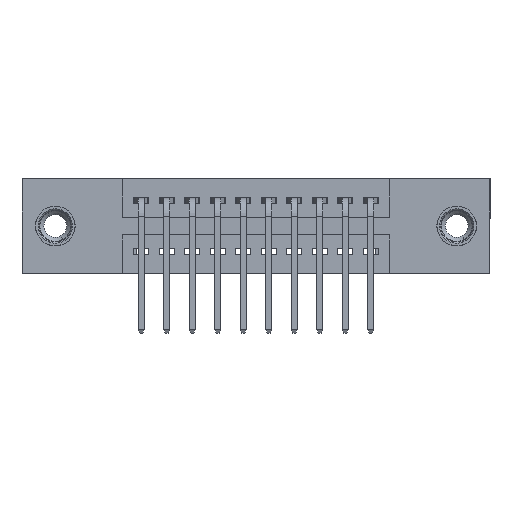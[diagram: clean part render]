
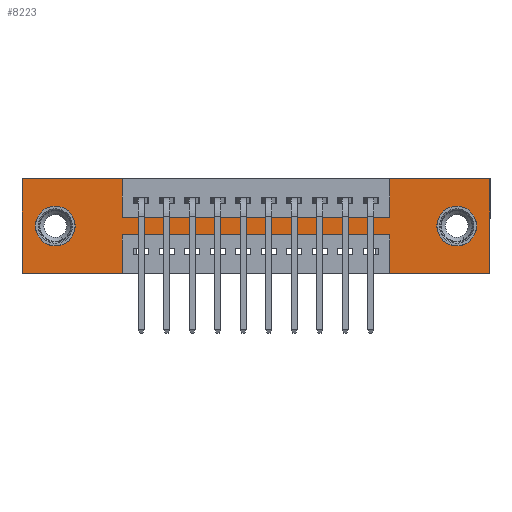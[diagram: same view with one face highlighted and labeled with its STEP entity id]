
A CAD part, front view. The second image highlights one B-rep face of the part: STEP entity #8223.
In plain terms, the highlighted planar face has unit normal (0, -1, 0).
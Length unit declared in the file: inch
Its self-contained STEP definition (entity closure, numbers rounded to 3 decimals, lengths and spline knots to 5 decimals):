
#67 = EDGE_CURVE ( 'NONE', #1339, #11391, #10440, .T. ) ;
#156 = CARTESIAN_POINT ( 'NONE',  ( 0.13, 0., -0.185 ) ) ;
#175 = LINE ( 'NONE', #6462, #6114 ) ;
#178 = CARTESIAN_POINT ( 'NONE',  ( 0.3925, 0., -0.15 ) ) ;
#489 = LINE ( 'NONE', #2541, #10583 ) ;
#529 = EDGE_CURVE ( 'NONE', #3014, #15972, #14744, .T. ) ;
#532 = CARTESIAN_POINT ( 'NONE',  ( 0.3925, 0., -0.37 ) ) ;
#799 = EDGE_LOOP ( 'NONE', ( #4511, #5727 ) ) ;
#966 = DIRECTION ( 'NONE',  ( 0., 0., 1. ) ) ;
#1264 = ORIENTED_EDGE ( 'NONE', *, *, #6913, .F. ) ;
#1339 = VERTEX_POINT ( 'NONE', #8443 ) ;
#1529 = DIRECTION ( 'NONE',  ( 0., 0., 1. ) ) ;
#1613 = CARTESIAN_POINT ( 'NONE',  ( 0., 0., 0. ) ) ;
#1901 = CARTESIAN_POINT ( 'NONE',  ( 1.4425, 0., -0.37 ) ) ;
#1910 = VERTEX_POINT ( 'NONE', #16460 ) ;
#1972 = EDGE_CURVE ( 'NONE', #15239, #2519, #2862, .T. ) ;
#2015 = CIRCLE ( 'NONE', #12170, 0.078 ) ;
#2458 = CARTESIAN_POINT ( 'NONE',  ( 0., 0., -0.37 ) ) ;
#2519 = VERTEX_POINT ( 'NONE', #4449 ) ;
#2522 = LINE ( 'NONE', #12769, #15750 ) ;
#2536 = CARTESIAN_POINT ( 'NONE',  ( 1.4425, 0., 0. ) ) ;
#2541 = CARTESIAN_POINT ( 'NONE',  ( 0.3925, 0., -0.15 ) ) ;
#2862 = LINE ( 'NONE', #7168, #9425 ) ;
#2865 = CARTESIAN_POINT ( 'NONE',  ( 1.705, 0., -0.107 ) ) ;
#2927 = LINE ( 'NONE', #9059, #9486 ) ;
#3014 = VERTEX_POINT ( 'NONE', #2458 ) ;
#3538 = CARTESIAN_POINT ( 'NONE',  ( 0.3925, 0., 0. ) ) ;
#3755 = EDGE_CURVE ( 'NONE', #11391, #9415, #10949, .T. ) ;
#4160 = VECTOR ( 'NONE', #13071, 39.37008 ) ;
#4161 = CARTESIAN_POINT ( 'NONE',  ( 0.3925, 0., -0.22 ) ) ;
#4449 = CARTESIAN_POINT ( 'NONE',  ( 1.835, 0., 0. ) ) ;
#4511 = ORIENTED_EDGE ( 'NONE', *, *, #8137, .T. ) ;
#4864 = CARTESIAN_POINT ( 'NONE',  ( 0., 0., -0.37 ) ) ;
#4930 = DIRECTION ( 'NONE',  ( 0., 0., -1. ) ) ;
#5026 = AXIS2_PLACEMENT_3D ( 'NONE', #156, #9443, #1529 ) ;
#5072 = VECTOR ( 'NONE', #5987, 39.37008 ) ;
#5142 = ORIENTED_EDGE ( 'NONE', *, *, #6101, .F. ) ;
#5353 = ORIENTED_EDGE ( 'NONE', *, *, #16474, .F. ) ;
#5378 = EDGE_LOOP ( 'NONE', ( #9885, #6919, #7741, #5142, #8521, #5543, #15941, #16689, #14219, #1264, #8336, #5353 ) ) ;
#5523 = ORIENTED_EDGE ( 'NONE', *, *, #10659, .T. ) ;
#5543 = ORIENTED_EDGE ( 'NONE', *, *, #1972, .F. ) ;
#5727 = ORIENTED_EDGE ( 'NONE', *, *, #14729, .T. ) ;
#5987 = DIRECTION ( 'NONE',  ( 0., 0., 1. ) ) ;
#6001 = CARTESIAN_POINT ( 'NONE',  ( 0.13, 0., -0.185 ) ) ;
#6031 = CIRCLE ( 'NONE', #13560, 0.078 ) ;
#6101 = EDGE_CURVE ( 'NONE', #10907, #1339, #16678, .T. ) ;
#6114 = VECTOR ( 'NONE', #9019, 39.37008 ) ;
#6422 = EDGE_CURVE ( 'NONE', #9415, #15403, #175, .T. ) ;
#6434 = CARTESIAN_POINT ( 'NONE',  ( 0.3925, 0., 0. ) ) ;
#6462 = CARTESIAN_POINT ( 'NONE',  ( 0.3925, 0., -0.37 ) ) ;
#6698 = CARTESIAN_POINT ( 'NONE',  ( 0., 0., 0. ) ) ;
#6738 = EDGE_CURVE ( 'NONE', #10102, #13054, #12222, .T. ) ;
#6744 = CARTESIAN_POINT ( 'NONE',  ( 1.705, 0., -0.185 ) ) ;
#6764 = CARTESIAN_POINT ( 'NONE',  ( 1.705, 0., -0.185 ) ) ;
#6913 = EDGE_CURVE ( 'NONE', #15972, #10102, #2927, .T. ) ;
#6919 = ORIENTED_EDGE ( 'NONE', *, *, #3755, .F. ) ;
#7036 = FACE_OUTER_BOUND ( 'NONE', #5378, .T. ) ;
#7079 = DIRECTION ( 'NONE',  ( -1., 0., 0. ) ) ;
#7083 = VECTOR ( 'NONE', #966, 39.37008 ) ;
#7168 = CARTESIAN_POINT ( 'NONE',  ( 0., 0., 0. ) ) ;
#7203 = VERTEX_POINT ( 'NONE', #9606 ) ;
#7281 = DIRECTION ( 'NONE',  ( 0., 0., 1. ) ) ;
#7375 = VERTEX_POINT ( 'NONE', #16220 ) ;
#7451 = DIRECTION ( 'NONE',  ( 0., 0., -1. ) ) ;
#7741 = ORIENTED_EDGE ( 'NONE', *, *, #67, .F. ) ;
#8038 = DIRECTION ( 'NONE',  ( 0., 0., -1. ) ) ;
#8056 = DIRECTION ( 'NONE',  ( 0., 0., -1. ) ) ;
#8137 = EDGE_CURVE ( 'NONE', #7375, #1910, #2015, .T. ) ;
#8223 = ADVANCED_FACE ( 'NONE', ( #14527, #13733, #7036 ), #12388, .T. ) ;
#8283 = CARTESIAN_POINT ( 'NONE',  ( 1.4425, 0., -0.22 ) ) ;
#8336 = ORIENTED_EDGE ( 'NONE', *, *, #529, .F. ) ;
#8443 = CARTESIAN_POINT ( 'NONE',  ( 1.4425, 0., -0.37 ) ) ;
#8453 = EDGE_CURVE ( 'NONE', #13054, #7203, #489, .T. ) ;
#8521 = ORIENTED_EDGE ( 'NONE', *, *, #12241, .F. ) ;
#8522 = EDGE_CURVE ( 'NONE', #8973, #16376, #6031, .T. ) ;
#8723 = VECTOR ( 'NONE', #14192, 39.37008 ) ;
#8835 = AXIS2_PLACEMENT_3D ( 'NONE', #6744, #15519, #8038 ) ;
#8892 = VECTOR ( 'NONE', #4930, 39.37008 ) ;
#8973 = VERTEX_POINT ( 'NONE', #13958 ) ;
#9019 = DIRECTION ( 'NONE',  ( 0., 0., -1. ) ) ;
#9059 = CARTESIAN_POINT ( 'NONE',  ( 0., 0., 0. ) ) ;
#9415 = VERTEX_POINT ( 'NONE', #12687 ) ;
#9425 = VECTOR ( 'NONE', #15916, 39.37008 ) ;
#9443 = DIRECTION ( 'NONE',  ( 0., 1., 0. ) ) ;
#9486 = VECTOR ( 'NONE', #14049, 39.37008 ) ;
#9540 = VECTOR ( 'NONE', #12276, 39.37008 ) ;
#9606 = CARTESIAN_POINT ( 'NONE',  ( 1.4425, 0., -0.15 ) ) ;
#9885 = ORIENTED_EDGE ( 'NONE', *, *, #6422, .F. ) ;
#9900 = LINE ( 'NONE', #2536, #8723 ) ;
#10102 = VERTEX_POINT ( 'NONE', #6434 ) ;
#10288 = DIRECTION ( 'NONE',  ( 0., 0., -1. ) ) ;
#10353 = DIRECTION ( 'NONE',  ( 1., 0., 0. ) ) ;
#10440 = LINE ( 'NONE', #1901, #7083 ) ;
#10569 = CIRCLE ( 'NONE', #5026, 0.078 ) ;
#10583 = VECTOR ( 'NONE', #10353, 39.37008 ) ;
#10659 = EDGE_CURVE ( 'NONE', #16376, #8973, #15230, .T. ) ;
#10907 = VERTEX_POINT ( 'NONE', #14773 ) ;
#10949 = LINE ( 'NONE', #4161, #4160 ) ;
#11391 = VERTEX_POINT ( 'NONE', #8283 ) ;
#11796 = EDGE_CURVE ( 'NONE', #7203, #15239, #9900, .T. ) ;
#12170 = AXIS2_PLACEMENT_3D ( 'NONE', #6001, #14812, #7281 ) ;
#12222 = LINE ( 'NONE', #3538, #8892 ) ;
#12241 = EDGE_CURVE ( 'NONE', #2519, #10907, #2522, .T. ) ;
#12276 = DIRECTION ( 'NONE',  ( -1., 0., 0. ) ) ;
#12388 = PLANE ( 'NONE',  #16315 ) ;
#12625 = ORIENTED_EDGE ( 'NONE', *, *, #8522, .T. ) ;
#12687 = CARTESIAN_POINT ( 'NONE',  ( 0.3925, 0., -0.22 ) ) ;
#12769 = CARTESIAN_POINT ( 'NONE',  ( 1.835, 0., 0. ) ) ;
#13054 = VERTEX_POINT ( 'NONE', #178 ) ;
#13071 = DIRECTION ( 'NONE',  ( -1., 0., 0. ) ) ;
#13437 = VECTOR ( 'NONE', #7079, 39.37008 ) ;
#13472 = EDGE_LOOP ( 'NONE', ( #5523, #12625 ) ) ;
#13558 = CARTESIAN_POINT ( 'NONE',  ( 0., 0., -0.37 ) ) ;
#13560 = AXIS2_PLACEMENT_3D ( 'NONE', #6764, #15539, #8056 ) ;
#13733 = FACE_BOUND ( 'NONE', #799, .T. ) ;
#13958 = CARTESIAN_POINT ( 'NONE',  ( 1.705, 0., -0.263 ) ) ;
#14049 = DIRECTION ( 'NONE',  ( 1., 0., 0. ) ) ;
#14192 = DIRECTION ( 'NONE',  ( 0., 0., 1. ) ) ;
#14219 = ORIENTED_EDGE ( 'NONE', *, *, #6738, .F. ) ;
#14527 = FACE_BOUND ( 'NONE', #13472, .T. ) ;
#14621 = CARTESIAN_POINT ( 'NONE',  ( 0., 0., -0.37 ) ) ;
#14729 = EDGE_CURVE ( 'NONE', #1910, #7375, #10569, .T. ) ;
#14744 = LINE ( 'NONE', #6698, #5072 ) ;
#14773 = CARTESIAN_POINT ( 'NONE',  ( 1.835, 0., -0.37 ) ) ;
#14812 = DIRECTION ( 'NONE',  ( 0., 1., 0. ) ) ;
#14958 = DIRECTION ( 'NONE',  ( 0., -1., 0. ) ) ;
#15230 = CIRCLE ( 'NONE', #8835, 0.078 ) ;
#15239 = VERTEX_POINT ( 'NONE', #15786 ) ;
#15403 = VERTEX_POINT ( 'NONE', #532 ) ;
#15519 = DIRECTION ( 'NONE',  ( 0., 1., 0. ) ) ;
#15539 = DIRECTION ( 'NONE',  ( 0., 1., 0. ) ) ;
#15750 = VECTOR ( 'NONE', #10288, 39.37008 ) ;
#15786 = CARTESIAN_POINT ( 'NONE',  ( 1.4425, 0., 0. ) ) ;
#15916 = DIRECTION ( 'NONE',  ( 1., 0., 0. ) ) ;
#15941 = ORIENTED_EDGE ( 'NONE', *, *, #11796, .F. ) ;
#15972 = VERTEX_POINT ( 'NONE', #1613 ) ;
#16145 = LINE ( 'NONE', #13558, #9540 ) ;
#16220 = CARTESIAN_POINT ( 'NONE',  ( 0.13, 0., -0.107 ) ) ;
#16315 = AXIS2_PLACEMENT_3D ( 'NONE', #4864, #14958, #7451 ) ;
#16376 = VERTEX_POINT ( 'NONE', #2865 ) ;
#16460 = CARTESIAN_POINT ( 'NONE',  ( 0.13, 0., -0.263 ) ) ;
#16474 = EDGE_CURVE ( 'NONE', #15403, #3014, #16145, .T. ) ;
#16678 = LINE ( 'NONE', #14621, #13437 ) ;
#16689 = ORIENTED_EDGE ( 'NONE', *, *, #8453, .F. ) ;
